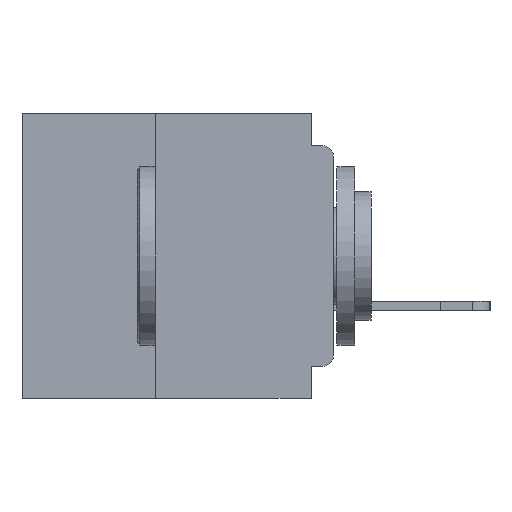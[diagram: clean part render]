
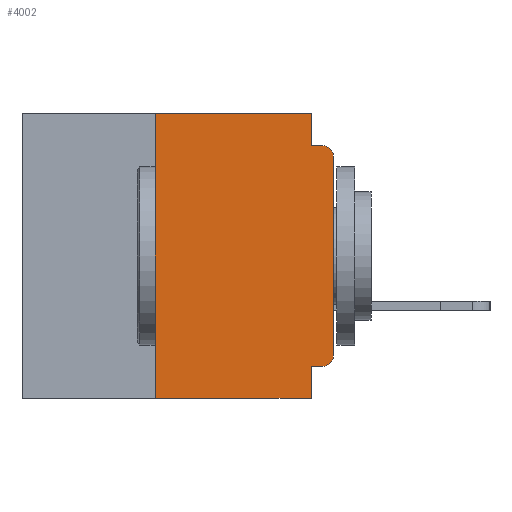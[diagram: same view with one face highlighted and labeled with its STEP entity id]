
A CAD part, left-side view. The second image highlights one B-rep face of the part: STEP entity #4002.
In plain terms, the highlighted planar face has unit normal (-1, 0, 0).
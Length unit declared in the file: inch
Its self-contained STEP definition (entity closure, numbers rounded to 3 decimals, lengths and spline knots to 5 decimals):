
#162 = AXIS2_PLACEMENT_3D ( 'NONE', #3856, #29944, #7638 ) ;
#1572 = DIRECTION ( 'NONE',  ( 0., 0., -1. ) ) ;
#2397 = EDGE_CURVE ( 'NONE', #16804, #19549, #34999, .T. ) ;
#2456 = LINE ( 'NONE', #40578, #42249 ) ;
#2512 = CARTESIAN_POINT ( 'NONE',  ( 0., 0.25, 0. ) ) ;
#2689 = DIRECTION ( 'NONE',  ( -1., 0., 0. ) ) ;
#3856 = CARTESIAN_POINT ( 'NONE',  ( 0., 0.015, -0.34 ) ) ;
#4002 = ADVANCED_FACE ( 'NONE', ( #19600 ), #5922, .F. ) ;
#4300 = VERTEX_POINT ( 'NONE', #19010 ) ;
#4706 = ORIENTED_EDGE ( 'NONE', *, *, #38467, .F. ) ;
#5168 = CARTESIAN_POINT ( 'NONE',  ( 0., 0.031, 0. ) ) ;
#5272 = ORIENTED_EDGE ( 'NONE', *, *, #19463, .T. ) ;
#5774 = EDGE_LOOP ( 'NONE', ( #45586, #5272, #38594, #13399, #4706, #7683, #30990, #25726, #39884, #20551 ) ) ;
#5810 = DIRECTION ( 'NONE',  ( 0., 0., -1. ) ) ;
#5871 = DIRECTION ( 'NONE',  ( 1., 0., 0. ) ) ;
#5922 = PLANE ( 'NONE',  #14824 ) ;
#6031 = CARTESIAN_POINT ( 'NONE',  ( 0., 0.437, 0. ) ) ;
#7638 = DIRECTION ( 'NONE',  ( 0., 0., -1. ) ) ;
#7683 = ORIENTED_EDGE ( 'NONE', *, *, #29110, .F. ) ;
#9162 = VECTOR ( 'NONE', #23768, 39.37008 ) ;
#9420 = CIRCLE ( 'NONE', #10683, 0.015 ) ;
#10683 = AXIS2_PLACEMENT_3D ( 'NONE', #25026, #2689, #28768 ) ;
#10688 = LINE ( 'NONE', #47628, #18288 ) ;
#11476 = LINE ( 'NONE', #19983, #9162 ) ;
#11754 = CARTESIAN_POINT ( 'NONE',  ( 0., 0.015, -0.355 ) ) ;
#12276 = LINE ( 'NONE', #43530, #38633 ) ;
#13399 = ORIENTED_EDGE ( 'NONE', *, *, #41668, .F. ) ;
#14758 = VECTOR ( 'NONE', #21949, 39.37008 ) ;
#14824 = AXIS2_PLACEMENT_3D ( 'NONE', #6031, #5871, #5810 ) ;
#15006 = CARTESIAN_POINT ( 'NONE',  ( 0., 0., -0.355 ) ) ;
#15164 = VERTEX_POINT ( 'NONE', #47909 ) ;
#15923 = LINE ( 'NONE', #29267, #14758 ) ;
#16136 = CARTESIAN_POINT ( 'NONE',  ( 0., 0.25, -0.4 ) ) ;
#16804 = VERTEX_POINT ( 'NONE', #22202 ) ;
#16899 = VECTOR ( 'NONE', #41216, 39.37008 ) ;
#16940 = CIRCLE ( 'NONE', #162, 0.015 ) ;
#17715 = DIRECTION ( 'NONE',  ( 0., -1., 0. ) ) ;
#18288 = VECTOR ( 'NONE', #17715, 39.37008 ) ;
#19010 = CARTESIAN_POINT ( 'NONE',  ( 0., 0.031, -0.355 ) ) ;
#19463 = EDGE_CURVE ( 'NONE', #28012, #19549, #9420, .T. ) ;
#19549 = VERTEX_POINT ( 'NONE', #21773 ) ;
#19600 = FACE_OUTER_BOUND ( 'NONE', #5774, .T. ) ;
#19983 = CARTESIAN_POINT ( 'NONE',  ( 0., 0., 0. ) ) ;
#20551 = ORIENTED_EDGE ( 'NONE', *, *, #33494, .T. ) ;
#21773 = CARTESIAN_POINT ( 'NONE',  ( 0., 0.015, -0.045 ) ) ;
#21891 = DIRECTION ( 'NONE',  ( 0., 0., 1. ) ) ;
#21949 = DIRECTION ( 'NONE',  ( 0., 0., -1. ) ) ;
#22202 = CARTESIAN_POINT ( 'NONE',  ( 0., 0.031, -0.045 ) ) ;
#23768 = DIRECTION ( 'NONE',  ( 0., 0., 1. ) ) ;
#23888 = VECTOR ( 'NONE', #40679, 39.37008 ) ;
#25026 = CARTESIAN_POINT ( 'NONE',  ( 0., 0.015, -0.06 ) ) ;
#25726 = ORIENTED_EDGE ( 'NONE', *, *, #31757, .F. ) ;
#26637 = VECTOR ( 'NONE', #1572, 39.37008 ) ;
#27589 = VERTEX_POINT ( 'NONE', #16136 ) ;
#27645 = CARTESIAN_POINT ( 'NONE',  ( 0., 0.031, 0. ) ) ;
#28012 = VERTEX_POINT ( 'NONE', #48318 ) ;
#28768 = DIRECTION ( 'NONE',  ( 0., 0., -1. ) ) ;
#29110 = EDGE_CURVE ( 'NONE', #27589, #38481, #2456, .T. ) ;
#29267 = CARTESIAN_POINT ( 'NONE',  ( 0., 0.031, -0.4 ) ) ;
#29944 = DIRECTION ( 'NONE',  ( -1., 0., 0. ) ) ;
#30990 = ORIENTED_EDGE ( 'NONE', *, *, #31691, .T. ) ;
#31691 = EDGE_CURVE ( 'NONE', #27589, #15164, #10688, .T. ) ;
#31757 = EDGE_CURVE ( 'NONE', #4300, #15164, #15923, .T. ) ;
#32198 = DIRECTION ( 'NONE',  ( 0., -1., 0. ) ) ;
#33494 = EDGE_CURVE ( 'NONE', #47773, #40426, #16940, .T. ) ;
#34648 = EDGE_CURVE ( 'NONE', #47773, #4300, #35612, .T. ) ;
#34999 = LINE ( 'NONE', #41912, #23888 ) ;
#35612 = LINE ( 'NONE', #15006, #16899 ) ;
#36974 = CARTESIAN_POINT ( 'NONE',  ( 0., 0., -0.34 ) ) ;
#37805 = LINE ( 'NONE', #5168, #26637 ) ;
#38467 = EDGE_CURVE ( 'NONE', #38481, #45541, #12276, .T. ) ;
#38481 = VERTEX_POINT ( 'NONE', #2512 ) ;
#38594 = ORIENTED_EDGE ( 'NONE', *, *, #2397, .F. ) ;
#38633 = VECTOR ( 'NONE', #32198, 39.37008 ) ;
#39884 = ORIENTED_EDGE ( 'NONE', *, *, #34648, .F. ) ;
#40426 = VERTEX_POINT ( 'NONE', #36974 ) ;
#40578 = CARTESIAN_POINT ( 'NONE',  ( 0., 0.25, -0.4 ) ) ;
#40679 = DIRECTION ( 'NONE',  ( 0., -1., 0. ) ) ;
#41216 = DIRECTION ( 'NONE',  ( 0., 1., 0. ) ) ;
#41625 = EDGE_CURVE ( 'NONE', #40426, #28012, #11476, .T. ) ;
#41668 = EDGE_CURVE ( 'NONE', #45541, #16804, #37805, .T. ) ;
#41912 = CARTESIAN_POINT ( 'NONE',  ( 0., 0., -0.045 ) ) ;
#42249 = VECTOR ( 'NONE', #21891, 39.37008 ) ;
#43530 = CARTESIAN_POINT ( 'NONE',  ( 0., 0.437, 0. ) ) ;
#45541 = VERTEX_POINT ( 'NONE', #27645 ) ;
#45586 = ORIENTED_EDGE ( 'NONE', *, *, #41625, .T. ) ;
#47628 = CARTESIAN_POINT ( 'NONE',  ( 0., 0.437, -0.4 ) ) ;
#47773 = VERTEX_POINT ( 'NONE', #11754 ) ;
#47909 = CARTESIAN_POINT ( 'NONE',  ( 0., 0.031, -0.4 ) ) ;
#48318 = CARTESIAN_POINT ( 'NONE',  ( 0., 0., -0.06 ) ) ;
